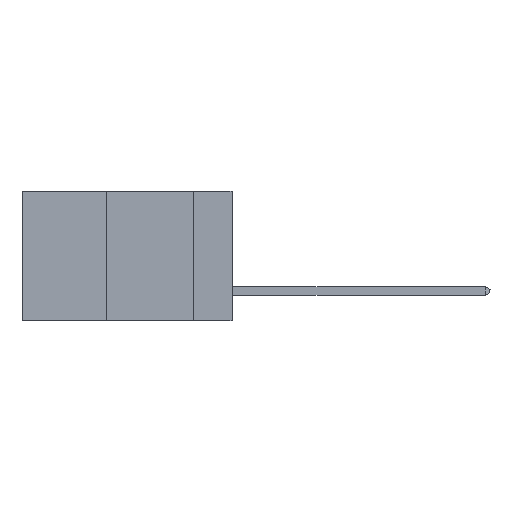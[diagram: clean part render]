
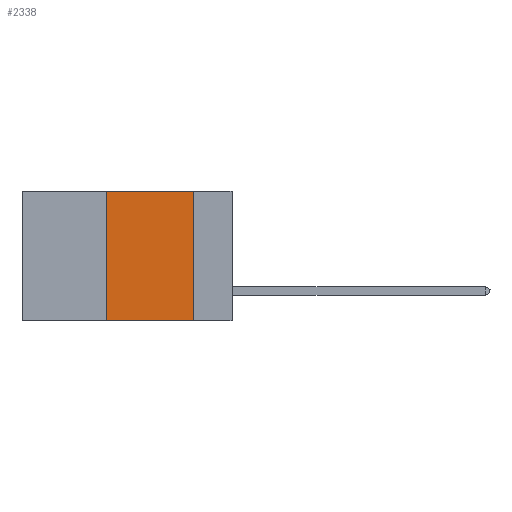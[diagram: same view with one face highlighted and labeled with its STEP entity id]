
A CAD part, left-side view. The second image highlights one B-rep face of the part: STEP entity #2338.
In plain terms, the highlighted planar face has unit normal (-1, 0, 0).
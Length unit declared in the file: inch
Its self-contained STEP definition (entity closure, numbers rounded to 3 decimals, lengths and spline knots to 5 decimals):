
#97 = CARTESIAN_POINT ( 'NONE',  ( 0., 0.11, -0.37 ) ) ;
#126 = LINE ( 'NONE', #5657, #3126 ) ;
#375 = VERTEX_POINT ( 'NONE', #11145 ) ;
#564 = DIRECTION ( 'NONE',  ( 1., 0., 0. ) ) ;
#830 = CARTESIAN_POINT ( 'NONE',  ( 0., 0.6, -0.37 ) ) ;
#1899 = EDGE_CURVE ( 'NONE', #8046, #10907, #9957, .T. ) ;
#2178 = CARTESIAN_POINT ( 'NONE',  ( 0., 0.36, 0. ) ) ;
#2299 = ORIENTED_EDGE ( 'NONE', *, *, #10149, .T. ) ;
#2309 = VECTOR ( 'NONE', #9310, 39.37008 ) ;
#2313 = ORIENTED_EDGE ( 'NONE', *, *, #1899, .F. ) ;
#2338 = ADVANCED_FACE ( 'NONE', ( #8838 ), #6615, .F. ) ;
#3126 = VECTOR ( 'NONE', #4760, 39.37008 ) ;
#4029 = CARTESIAN_POINT ( 'NONE',  ( 0., 0.36, 0. ) ) ;
#4239 = CARTESIAN_POINT ( 'NONE',  ( 0., 0.6, 0. ) ) ;
#4280 = DIRECTION ( 'NONE',  ( 0., -1., 0. ) ) ;
#4422 = DIRECTION ( 'NONE',  ( 0., -1., 0. ) ) ;
#4609 = VECTOR ( 'NONE', #4280, 39.37008 ) ;
#4760 = DIRECTION ( 'NONE',  ( 0., 0., -1. ) ) ;
#4784 = VECTOR ( 'NONE', #4422, 39.37008 ) ;
#4796 = EDGE_CURVE ( 'NONE', #375, #8046, #8743, .T. ) ;
#5504 = CARTESIAN_POINT ( 'NONE',  ( 0., 0.11, 0. ) ) ;
#5657 = CARTESIAN_POINT ( 'NONE',  ( 0., 0.11, 0. ) ) ;
#6615 = PLANE ( 'NONE',  #9897 ) ;
#6811 = ORIENTED_EDGE ( 'NONE', *, *, #4796, .F. ) ;
#7526 = ORIENTED_EDGE ( 'NONE', *, *, #9465, .F. ) ;
#7609 = DIRECTION ( 'NONE',  ( 0., 0., -1. ) ) ;
#8046 = VERTEX_POINT ( 'NONE', #2178 ) ;
#8656 = EDGE_LOOP ( 'NONE', ( #7526, #2313, #6811, #2299 ) ) ;
#8743 = LINE ( 'NONE', #4029, #2309 ) ;
#8838 = FACE_OUTER_BOUND ( 'NONE', #8656, .T. ) ;
#9310 = DIRECTION ( 'NONE',  ( 0., 0., 1. ) ) ;
#9465 = EDGE_CURVE ( 'NONE', #10907, #11264, #126, .T. ) ;
#9897 = AXIS2_PLACEMENT_3D ( 'NONE', #10165, #564, #7609 ) ;
#9957 = LINE ( 'NONE', #4239, #4609 ) ;
#10009 = LINE ( 'NONE', #830, #4784 ) ;
#10149 = EDGE_CURVE ( 'NONE', #375, #11264, #10009, .T. ) ;
#10165 = CARTESIAN_POINT ( 'NONE',  ( 0., 0.6, 0. ) ) ;
#10907 = VERTEX_POINT ( 'NONE', #5504 ) ;
#11145 = CARTESIAN_POINT ( 'NONE',  ( 0., 0.36, -0.37 ) ) ;
#11264 = VERTEX_POINT ( 'NONE', #97 ) ;
